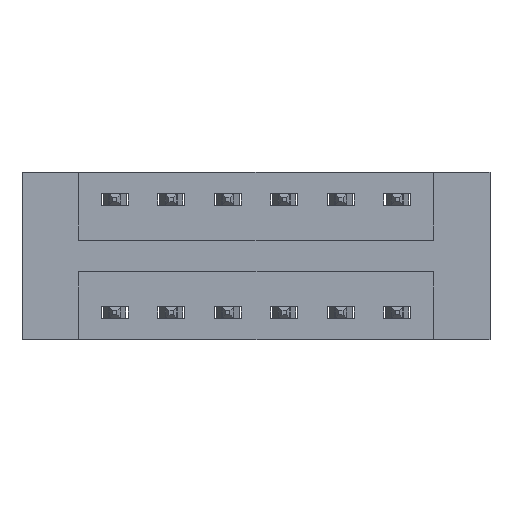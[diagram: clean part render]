
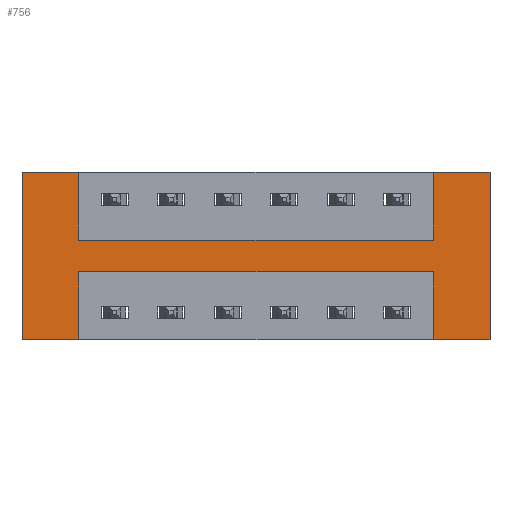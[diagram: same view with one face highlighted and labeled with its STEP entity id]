
A CAD part, front view. The second image highlights one B-rep face of the part: STEP entity #756.
In plain terms, the highlighted planar face has unit normal (0, -1, 0).
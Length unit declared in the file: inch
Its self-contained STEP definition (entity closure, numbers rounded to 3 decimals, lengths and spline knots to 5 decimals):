
#40 = VECTOR ( 'NONE', #1584, 39.37008 ) ;
#51 = CARTESIAN_POINT ( 'NONE',  ( 0.2625, 0., 0. ) ) ;
#61 = ORIENTED_EDGE ( 'NONE', *, *, #3543, .F. ) ;
#76 = EDGE_CURVE ( 'NONE', #1841, #3730, #1724, .T. ) ;
#133 = CARTESIAN_POINT ( 'NONE',  ( 0.3875, 0., -0.37 ) ) ;
#155 = CARTESIAN_POINT ( 'NONE',  ( 0., 0., 0. ) ) ;
#178 = VERTEX_POINT ( 'NONE', #5264 ) ;
#187 = CARTESIAN_POINT ( 'NONE',  ( 0.3875, 0., -0.22 ) ) ;
#201 = CARTESIAN_POINT ( 'NONE',  ( 0., 0., -0.37 ) ) ;
#299 = VECTOR ( 'NONE', #7404, 39.37008 ) ;
#457 = EDGE_CURVE ( 'NONE', #7779, #1185, #5228, .T. ) ;
#594 = CARTESIAN_POINT ( 'NONE',  ( 1.1725, 0., -0.15 ) ) ;
#631 = LINE ( 'NONE', #1299, #7448 ) ;
#687 = VECTOR ( 'NONE', #5502, 39.37008 ) ;
#750 = DIRECTION ( 'NONE',  ( 0., 0., -1. ) ) ;
#756 = ADVANCED_FACE ( 'NONE', ( #1157 ), #5667, .T. ) ;
#769 = EDGE_CURVE ( 'NONE', #4564, #5922, #4286, .T. ) ;
#830 = VERTEX_POINT ( 'NONE', #594 ) ;
#1157 = FACE_OUTER_BOUND ( 'NONE', #4062, .T. ) ;
#1185 = VERTEX_POINT ( 'NONE', #1399 ) ;
#1299 = CARTESIAN_POINT ( 'NONE',  ( 0.3875, 0., -0.15 ) ) ;
#1353 = CARTESIAN_POINT ( 'NONE',  ( 0.3875, 0., -0.37 ) ) ;
#1399 = CARTESIAN_POINT ( 'NONE',  ( 1.2975, 0., 0. ) ) ;
#1535 = LINE ( 'NONE', #155, #6590 ) ;
#1549 = CARTESIAN_POINT ( 'NONE',  ( 0., 0., 0. ) ) ;
#1584 = DIRECTION ( 'NONE',  ( 0., 0., 1. ) ) ;
#1681 = CARTESIAN_POINT ( 'NONE',  ( 1.2975, 0., 0. ) ) ;
#1724 = LINE ( 'NONE', #201, #8176 ) ;
#1841 = VERTEX_POINT ( 'NONE', #1353 ) ;
#1990 = DIRECTION ( 'NONE',  ( -1., 0., 0. ) ) ;
#2022 = CARTESIAN_POINT ( 'NONE',  ( 1.1725, 0., 0. ) ) ;
#2079 = EDGE_CURVE ( 'NONE', #178, #4564, #2727, .T. ) ;
#2193 = LINE ( 'NONE', #133, #299 ) ;
#2348 = CARTESIAN_POINT ( 'NONE',  ( 1.2975, 0., -0.37 ) ) ;
#2644 = LINE ( 'NONE', #2022, #5935 ) ;
#2650 = CARTESIAN_POINT ( 'NONE',  ( 0.2625, 0., 0. ) ) ;
#2727 = LINE ( 'NONE', #3527, #6014 ) ;
#2872 = CARTESIAN_POINT ( 'NONE',  ( 0.3875, 0., 0. ) ) ;
#2879 = ORIENTED_EDGE ( 'NONE', *, *, #5454, .F. ) ;
#2896 = DIRECTION ( 'NONE',  ( 0., 0., 1. ) ) ;
#2908 = VECTOR ( 'NONE', #7999, 39.37008 ) ;
#3196 = CARTESIAN_POINT ( 'NONE',  ( 0.2625, 0., -0.37 ) ) ;
#3449 = EDGE_CURVE ( 'NONE', #6594, #3730, #3708, .T. ) ;
#3481 = DIRECTION ( 'NONE',  ( 0., 0., -1. ) ) ;
#3527 = CARTESIAN_POINT ( 'NONE',  ( 1.1725, 0., -0.37 ) ) ;
#3543 = EDGE_CURVE ( 'NONE', #4613, #1185, #4662, .T. ) ;
#3570 = ORIENTED_EDGE ( 'NONE', *, *, #4709, .F. ) ;
#3680 = ORIENTED_EDGE ( 'NONE', *, *, #769, .F. ) ;
#3708 = LINE ( 'NONE', #51, #6968 ) ;
#3730 = VERTEX_POINT ( 'NONE', #3196 ) ;
#4062 = EDGE_LOOP ( 'NONE', ( #7013, #61, #3570, #6441, #2879, #8339, #6540, #7081, #5542, #3680, #8399, #5497 ) ) ;
#4286 = LINE ( 'NONE', #187, #687 ) ;
#4564 = VERTEX_POINT ( 'NONE', #5851 ) ;
#4572 = CARTESIAN_POINT ( 'NONE',  ( 0.3875, 0., 0. ) ) ;
#4613 = VERTEX_POINT ( 'NONE', #5882 ) ;
#4631 = VERTEX_POINT ( 'NONE', #4572 ) ;
#4637 = VERTEX_POINT ( 'NONE', #8364 ) ;
#4662 = LINE ( 'NONE', #1549, #2908 ) ;
#4709 = EDGE_CURVE ( 'NONE', #830, #4613, #2644, .T. ) ;
#4793 = DIRECTION ( 'NONE',  ( 0., -1., 0. ) ) ;
#5008 = VECTOR ( 'NONE', #6799, 39.37008 ) ;
#5228 = LINE ( 'NONE', #1681, #40 ) ;
#5264 = CARTESIAN_POINT ( 'NONE',  ( 1.1725, 0., -0.37 ) ) ;
#5454 = EDGE_CURVE ( 'NONE', #4631, #4637, #6719, .T. ) ;
#5497 = ORIENTED_EDGE ( 'NONE', *, *, #6001, .F. ) ;
#5502 = DIRECTION ( 'NONE',  ( -1., 0., 0. ) ) ;
#5542 = ORIENTED_EDGE ( 'NONE', *, *, #7651, .F. ) ;
#5560 = DIRECTION ( 'NONE',  ( 1., 0., 0. ) ) ;
#5667 = PLANE ( 'NONE',  #6833 ) ;
#5851 = CARTESIAN_POINT ( 'NONE',  ( 1.1725, 0., -0.22 ) ) ;
#5882 = CARTESIAN_POINT ( 'NONE',  ( 1.1725, 0., 0. ) ) ;
#5922 = VERTEX_POINT ( 'NONE', #7745 ) ;
#5935 = VECTOR ( 'NONE', #7823, 39.37008 ) ;
#6001 = EDGE_CURVE ( 'NONE', #7779, #178, #8337, .T. ) ;
#6014 = VECTOR ( 'NONE', #2896, 39.37008 ) ;
#6441 = ORIENTED_EDGE ( 'NONE', *, *, #7383, .F. ) ;
#6514 = VECTOR ( 'NONE', #8452, 39.37008 ) ;
#6540 = ORIENTED_EDGE ( 'NONE', *, *, #3449, .T. ) ;
#6556 = DIRECTION ( 'NONE',  ( 1., 0., 0. ) ) ;
#6590 = VECTOR ( 'NONE', #5560, 39.37008 ) ;
#6594 = VERTEX_POINT ( 'NONE', #2650 ) ;
#6609 = CARTESIAN_POINT ( 'NONE',  ( 0., 0., -0.37 ) ) ;
#6719 = LINE ( 'NONE', #2872, #5008 ) ;
#6799 = DIRECTION ( 'NONE',  ( 0., 0., -1. ) ) ;
#6833 = AXIS2_PLACEMENT_3D ( 'NONE', #7894, #4793, #3481 ) ;
#6968 = VECTOR ( 'NONE', #750, 39.37008 ) ;
#7013 = ORIENTED_EDGE ( 'NONE', *, *, #457, .T. ) ;
#7081 = ORIENTED_EDGE ( 'NONE', *, *, #76, .F. ) ;
#7383 = EDGE_CURVE ( 'NONE', #4637, #830, #631, .T. ) ;
#7404 = DIRECTION ( 'NONE',  ( 0., 0., -1. ) ) ;
#7448 = VECTOR ( 'NONE', #6556, 39.37008 ) ;
#7651 = EDGE_CURVE ( 'NONE', #5922, #1841, #2193, .T. ) ;
#7745 = CARTESIAN_POINT ( 'NONE',  ( 0.3875, 0., -0.22 ) ) ;
#7779 = VERTEX_POINT ( 'NONE', #2348 ) ;
#7823 = DIRECTION ( 'NONE',  ( 0., 0., 1. ) ) ;
#7894 = CARTESIAN_POINT ( 'NONE',  ( 0., 0., -0.37 ) ) ;
#7999 = DIRECTION ( 'NONE',  ( 1., 0., 0. ) ) ;
#8176 = VECTOR ( 'NONE', #1990, 39.37008 ) ;
#8337 = LINE ( 'NONE', #6609, #6514 ) ;
#8339 = ORIENTED_EDGE ( 'NONE', *, *, #8515, .F. ) ;
#8364 = CARTESIAN_POINT ( 'NONE',  ( 0.3875, 0., -0.15 ) ) ;
#8399 = ORIENTED_EDGE ( 'NONE', *, *, #2079, .F. ) ;
#8452 = DIRECTION ( 'NONE',  ( -1., 0., 0. ) ) ;
#8515 = EDGE_CURVE ( 'NONE', #6594, #4631, #1535, .T. ) ;
